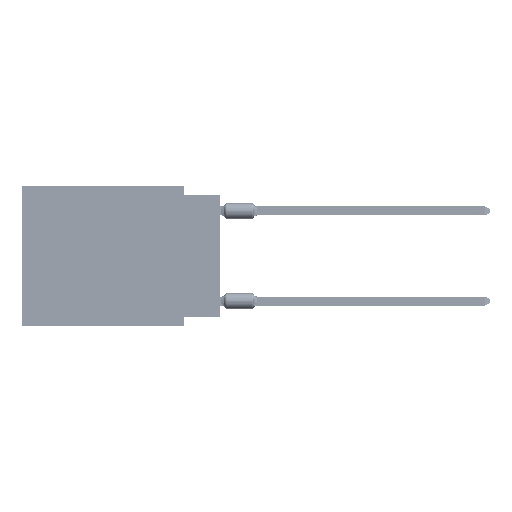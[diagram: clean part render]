
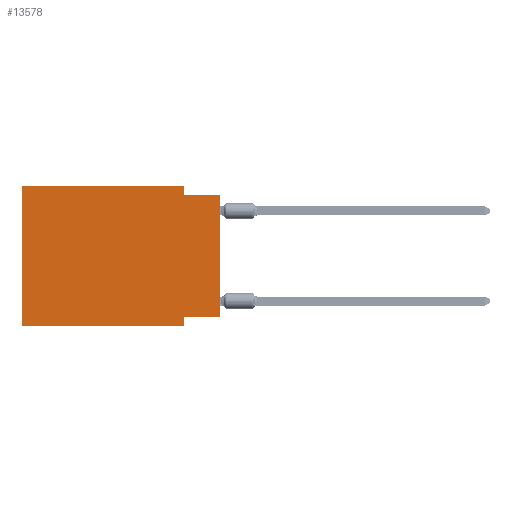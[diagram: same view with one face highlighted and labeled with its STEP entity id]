
A CAD part, left-side view. The second image highlights one B-rep face of the part: STEP entity #13578.
In plain terms, the highlighted planar face has unit normal (-1, 0, 0).
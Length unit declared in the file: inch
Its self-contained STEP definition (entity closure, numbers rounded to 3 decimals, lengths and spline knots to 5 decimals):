
#1 = CARTESIAN_POINT ( 'NONE',  ( 0., 0.1, 0. ) ) ;
#2325 = CARTESIAN_POINT ( 'NONE',  ( 0., 0., -0.025 ) ) ;
#2572 = ORIENTED_EDGE ( 'NONE', *, *, #29966, .F. ) ;
#3061 = DIRECTION ( 'NONE',  ( 0., 0., 1. ) ) ;
#3325 = CARTESIAN_POINT ( 'NONE',  ( 0., 0.55, -0.39 ) ) ;
#6147 = VERTEX_POINT ( 'NONE', #74328 ) ;
#7226 = DIRECTION ( 'NONE',  ( 0., 0., -1. ) ) ;
#7322 = ORIENTED_EDGE ( 'NONE', *, *, #22775, .F. ) ;
#7404 = EDGE_CURVE ( 'NONE', #14693, #69454, #58510, .T. ) ;
#7839 = CARTESIAN_POINT ( 'NONE',  ( 0., 0.55, 0. ) ) ;
#9563 = VECTOR ( 'NONE', #7226, 39.37008 ) ;
#9741 = CARTESIAN_POINT ( 'NONE',  ( 0., 0.55, 0. ) ) ;
#10469 = VECTOR ( 'NONE', #75813, 39.37008 ) ;
#12757 = VERTEX_POINT ( 'NONE', #23384 ) ;
#13578 = ADVANCED_FACE ( 'NONE', ( #40332 ), #66399, .F. ) ;
#14693 = VERTEX_POINT ( 'NONE', #31727 ) ;
#16952 = ORIENTED_EDGE ( 'NONE', *, *, #31551, .T. ) ;
#17855 = ORIENTED_EDGE ( 'NONE', *, *, #44979, .F. ) ;
#19799 = ORIENTED_EDGE ( 'NONE', *, *, #64297, .T. ) ;
#21723 = LINE ( 'NONE', #3325, #74915 ) ;
#22775 = EDGE_CURVE ( 'NONE', #32748, #14693, #57634, .T. ) ;
#23192 = VECTOR ( 'NONE', #50802, 39.37008 ) ;
#23384 = CARTESIAN_POINT ( 'NONE',  ( 0., 0.55, -0.39 ) ) ;
#24738 = CARTESIAN_POINT ( 'NONE',  ( 0., 0.55, 0. ) ) ;
#25494 = DIRECTION ( 'NONE',  ( 0., 1., 0. ) ) ;
#26949 = VECTOR ( 'NONE', #25494, 39.37008 ) ;
#29966 = EDGE_CURVE ( 'NONE', #6147, #72905, #31923, .T. ) ;
#31551 = EDGE_CURVE ( 'NONE', #12757, #49159, #21723, .T. ) ;
#31727 = CARTESIAN_POINT ( 'NONE',  ( 0., 0.1, 0. ) ) ;
#31923 = LINE ( 'NONE', #70833, #26949 ) ;
#32748 = VERTEX_POINT ( 'NONE', #9741 ) ;
#35568 = LINE ( 'NONE', #68461, #61888 ) ;
#37232 = LINE ( 'NONE', #45326, #60538 ) ;
#40332 = FACE_OUTER_BOUND ( 'NONE', #76949, .T. ) ;
#41004 = CARTESIAN_POINT ( 'NONE',  ( 0., 0.1, -0.365 ) ) ;
#44576 = CARTESIAN_POINT ( 'NONE',  ( 0., 0.55, 0. ) ) ;
#44979 = EDGE_CURVE ( 'NONE', #72905, #49159, #37232, .T. ) ;
#45326 = CARTESIAN_POINT ( 'NONE',  ( 0., 0.1, -0.39 ) ) ;
#49159 = VERTEX_POINT ( 'NONE', #53114 ) ;
#50802 = DIRECTION ( 'NONE',  ( 0., -1., 0. ) ) ;
#53114 = CARTESIAN_POINT ( 'NONE',  ( 0., 0.1, -0.39 ) ) ;
#54343 = LINE ( 'NONE', #54757, #77434 ) ;
#54757 = CARTESIAN_POINT ( 'NONE',  ( 0., 0., 0. ) ) ;
#55195 = DIRECTION ( 'NONE',  ( 0., -1., 0. ) ) ;
#56453 = DIRECTION ( 'NONE',  ( 0., 0., -1. ) ) ;
#56637 = CARTESIAN_POINT ( 'NONE',  ( 0., 0.1, -0.025 ) ) ;
#57634 = LINE ( 'NONE', #24738, #23192 ) ;
#58510 = LINE ( 'NONE', #1, #9563 ) ;
#59977 = DIRECTION ( 'NONE',  ( 1., 0., 0. ) ) ;
#60538 = VECTOR ( 'NONE', #56453, 39.37008 ) ;
#61888 = VECTOR ( 'NONE', #55195, 39.37008 ) ;
#63405 = LINE ( 'NONE', #44576, #10469 ) ;
#64297 = EDGE_CURVE ( 'NONE', #6147, #69665, #54343, .T. ) ;
#66399 = PLANE ( 'NONE',  #81137 ) ;
#66895 = ORIENTED_EDGE ( 'NONE', *, *, #79796, .F. ) ;
#67027 = DIRECTION ( 'NONE',  ( 0., -1., 0. ) ) ;
#68461 = CARTESIAN_POINT ( 'NONE',  ( 0., 0., -0.025 ) ) ;
#69454 = VERTEX_POINT ( 'NONE', #56637 ) ;
#69665 = VERTEX_POINT ( 'NONE', #2325 ) ;
#70833 = CARTESIAN_POINT ( 'NONE',  ( 0., 0., -0.365 ) ) ;
#71126 = ORIENTED_EDGE ( 'NONE', *, *, #7404, .F. ) ;
#72905 = VERTEX_POINT ( 'NONE', #41004 ) ;
#74328 = CARTESIAN_POINT ( 'NONE',  ( 0., 0., -0.365 ) ) ;
#74915 = VECTOR ( 'NONE', #67027, 39.37008 ) ;
#75813 = DIRECTION ( 'NONE',  ( 0., 0., 1. ) ) ;
#76949 = EDGE_LOOP ( 'NONE', ( #19799, #81757, #71126, #7322, #66895, #16952, #17855, #2572 ) ) ;
#77039 = EDGE_CURVE ( 'NONE', #69454, #69665, #35568, .T. ) ;
#77434 = VECTOR ( 'NONE', #3061, 39.37008 ) ;
#79648 = DIRECTION ( 'NONE',  ( 0., 0., -1. ) ) ;
#79796 = EDGE_CURVE ( 'NONE', #12757, #32748, #63405, .T. ) ;
#81137 = AXIS2_PLACEMENT_3D ( 'NONE', #7839, #59977, #79648 ) ;
#81757 = ORIENTED_EDGE ( 'NONE', *, *, #77039, .F. ) ;
